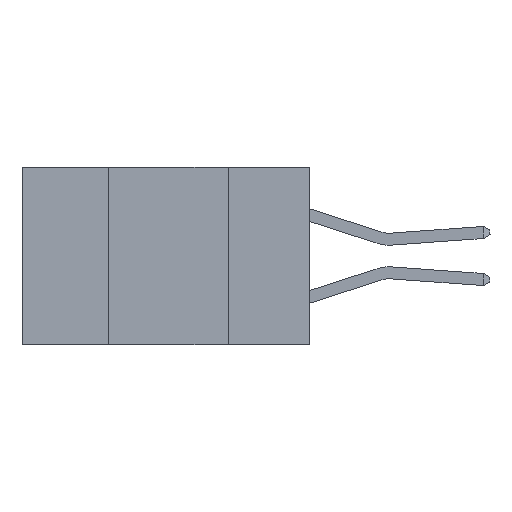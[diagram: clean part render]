
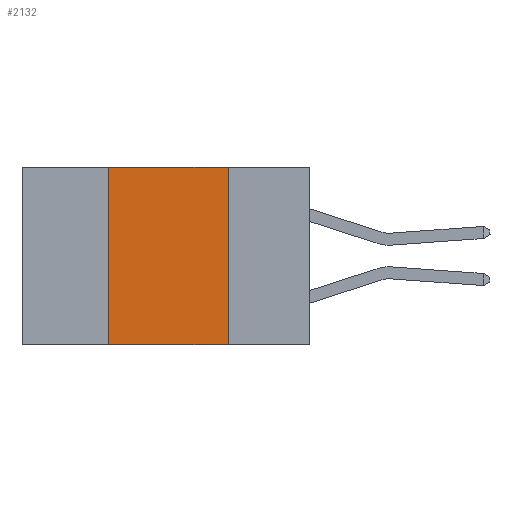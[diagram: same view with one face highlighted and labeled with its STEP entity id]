
A CAD part, left-side view. The second image highlights one B-rep face of the part: STEP entity #2132.
In plain terms, the highlighted planar face has unit normal (-1, 0, 0).
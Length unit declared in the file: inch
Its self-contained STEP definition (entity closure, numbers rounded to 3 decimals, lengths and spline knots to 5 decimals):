
#5 = LINE ( 'NONE', #5756, #8396 ) ;
#143 = EDGE_LOOP ( 'NONE', ( #8244, #6847, #3241, #2818 ) ) ;
#301 = VECTOR ( 'NONE', #1207, 39.37008 ) ;
#412 = EDGE_CURVE ( 'NONE', #8618, #10458, #10658, .T. ) ;
#606 = CARTESIAN_POINT ( 'NONE',  ( 0., 0.17, -0.37 ) ) ;
#900 = VERTEX_POINT ( 'NONE', #6833 ) ;
#1207 = DIRECTION ( 'NONE',  ( 0., -1., 0. ) ) ;
#2132 = ADVANCED_FACE ( 'NONE', ( #4113 ), #10676, .F. ) ;
#2818 = ORIENTED_EDGE ( 'NONE', *, *, #412, .T. ) ;
#3241 = ORIENTED_EDGE ( 'NONE', *, *, #6522, .F. ) ;
#3780 = CARTESIAN_POINT ( 'NONE',  ( 0., 0.42, 0. ) ) ;
#3972 = CARTESIAN_POINT ( 'NONE',  ( 0., 0.6, -0.37 ) ) ;
#4113 = FACE_OUTER_BOUND ( 'NONE', #143, .T. ) ;
#4379 = LINE ( 'NONE', #9018, #10792 ) ;
#4475 = DIRECTION ( 'NONE',  ( 0., 0., -1. ) ) ;
#4758 = AXIS2_PLACEMENT_3D ( 'NONE', #5917, #4990, #11743 ) ;
#4990 = DIRECTION ( 'NONE',  ( 1., 0., 0. ) ) ;
#5416 = LINE ( 'NONE', #9253, #10307 ) ;
#5756 = CARTESIAN_POINT ( 'NONE',  ( 0., 0.42, -0.37 ) ) ;
#5917 = CARTESIAN_POINT ( 'NONE',  ( 0., 0.6, 0. ) ) ;
#6130 = DIRECTION ( 'NONE',  ( 0., -1., 0. ) ) ;
#6401 = EDGE_CURVE ( 'NONE', #9103, #900, #4379, .T. ) ;
#6522 = EDGE_CURVE ( 'NONE', #8618, #9103, #5, .T. ) ;
#6833 = CARTESIAN_POINT ( 'NONE',  ( 0., 0.17, 0. ) ) ;
#6847 = ORIENTED_EDGE ( 'NONE', *, *, #6401, .F. ) ;
#8061 = CARTESIAN_POINT ( 'NONE',  ( 0., 0.42, -0.37 ) ) ;
#8244 = ORIENTED_EDGE ( 'NONE', *, *, #11086, .F. ) ;
#8396 = VECTOR ( 'NONE', #9594, 39.37008 ) ;
#8618 = VERTEX_POINT ( 'NONE', #8061 ) ;
#9018 = CARTESIAN_POINT ( 'NONE',  ( 0., 0.6, 0. ) ) ;
#9103 = VERTEX_POINT ( 'NONE', #3780 ) ;
#9253 = CARTESIAN_POINT ( 'NONE',  ( 0., 0.17, -0.37 ) ) ;
#9594 = DIRECTION ( 'NONE',  ( 0., 0., 1. ) ) ;
#10307 = VECTOR ( 'NONE', #4475, 39.37008 ) ;
#10458 = VERTEX_POINT ( 'NONE', #606 ) ;
#10658 = LINE ( 'NONE', #3972, #301 ) ;
#10676 = PLANE ( 'NONE',  #4758 ) ;
#10792 = VECTOR ( 'NONE', #6130, 39.37008 ) ;
#11086 = EDGE_CURVE ( 'NONE', #900, #10458, #5416, .T. ) ;
#11743 = DIRECTION ( 'NONE',  ( 0., 0., -1. ) ) ;
